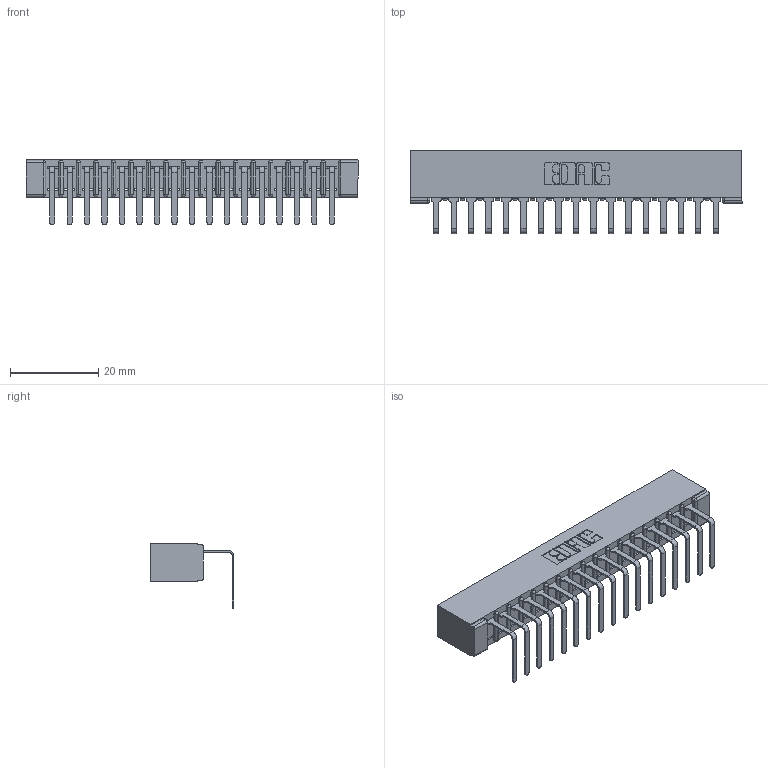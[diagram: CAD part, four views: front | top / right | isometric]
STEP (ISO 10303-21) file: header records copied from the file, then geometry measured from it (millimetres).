
FILE_DESCRIPTION (( 'STEP AP203' ), '1' );
FILE_NAME ('307-017-558-101.STEP', '2019-09-04T12:55:10', ( '' ), ( '' ), 'SwSTEP 2.0', 'SolidWorks 2016', '' );
FILE_SCHEMA (( 'CONFIG_CONTROL_DESIGN' ));
Length unit declared in the file: inch
Products named in the file (3): 307 Part_No Mounting Lugs; 307-017-558-101; 307-290-001_558 - 2 (Single)
Assembly tree (18 placements, depth 2):
  307-017-558-101
    307 Part_No Mounting Lugs
    307-290-001_558 - 2 (Single)  x17
Bounding box: 75.23 x 18.96 x 14.81 mm (x, y, z)
Volume: 5038.2 mm3; surface area: 8402.1 mm2
Topology: 18 solids, 18 shells, 1148 faces, 3257 edges, 2098 vertices
Faces by surface type: plane 729, cylinder 383, sphere 36
Entity records: 17482 total; most frequent: CARTESIAN_POINT 2936, ORIENTED_EDGE 2922, DIRECTION 2869, EDGE_CURVE 1461, VECTOR 1111, LINE 1111, VERTEX_POINT 946, AXIS2_PLACEMENT_3D 879
